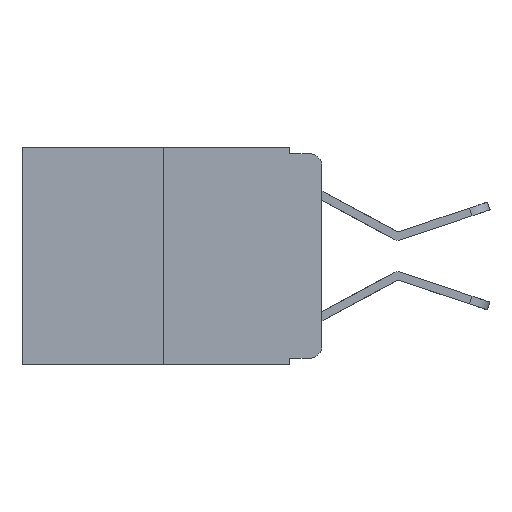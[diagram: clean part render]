
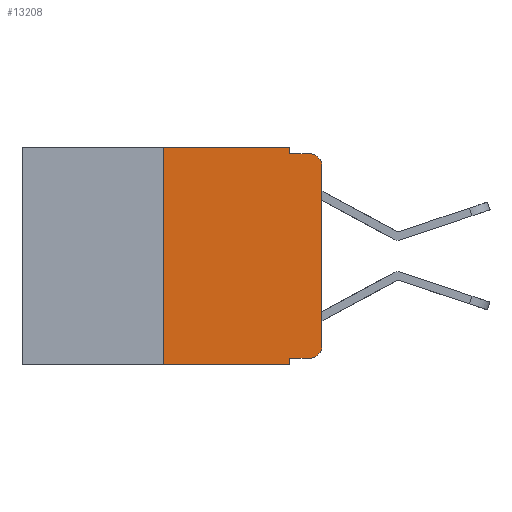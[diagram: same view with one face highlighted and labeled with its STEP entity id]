
A CAD part, left-side view. The second image highlights one B-rep face of the part: STEP entity #13208.
In plain terms, the highlighted planar face has unit normal (-1, 0, 0).
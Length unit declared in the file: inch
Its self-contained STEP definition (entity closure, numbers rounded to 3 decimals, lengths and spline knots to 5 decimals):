
#292 = ORIENTED_EDGE ( 'NONE', *, *, #13894, .F. ) ;
#390 = ORIENTED_EDGE ( 'NONE', *, *, #7782, .F. ) ;
#417 = ORIENTED_EDGE ( 'NONE', *, *, #17921, .T. ) ;
#485 = EDGE_CURVE ( 'NONE', #21264, #4814, #18064, .T. ) ;
#615 = VERTEX_POINT ( 'NONE', #5662 ) ;
#656 = ORIENTED_EDGE ( 'NONE', *, *, #8458, .F. ) ;
#931 = ORIENTED_EDGE ( 'NONE', *, *, #13237, .T. ) ;
#1133 = ORIENTED_EDGE ( 'NONE', *, *, #14154, .T. ) ;
#1221 = CARTESIAN_POINT ( 'NONE',  ( 0., 0.051, 0. ) ) ;
#1790 = AXIS2_PLACEMENT_3D ( 'NONE', #21017, #22693, #12442 ) ;
#2710 = CARTESIAN_POINT ( 'NONE',  ( 0., 0.051, -0.333 ) ) ;
#2815 = DIRECTION ( 'NONE',  ( 0., 0., -1. ) ) ;
#2845 = CARTESIAN_POINT ( 'NONE',  ( 0., 0., 0. ) ) ;
#3142 = CARTESIAN_POINT ( 'NONE',  ( 0., 0.02, -0.01 ) ) ;
#3292 = VERTEX_POINT ( 'NONE', #4111 ) ;
#3741 = ORIENTED_EDGE ( 'NONE', *, *, #21309, .F. ) ;
#4111 = CARTESIAN_POINT ( 'NONE',  ( 0., 0.25, -0.343 ) ) ;
#4673 = VECTOR ( 'NONE', #13669, 39.37008 ) ;
#4814 = VERTEX_POINT ( 'NONE', #3142 ) ;
#4934 = VECTOR ( 'NONE', #2815, 39.37008 ) ;
#5662 = CARTESIAN_POINT ( 'NONE',  ( 0., 0., -0.313 ) ) ;
#5788 = CARTESIAN_POINT ( 'NONE',  ( 0., 0.02, -0.313 ) ) ;
#6361 = DIRECTION ( 'NONE',  ( 0., -1., 0. ) ) ;
#6929 = CARTESIAN_POINT ( 'NONE',  ( 0., 0.473, 0. ) ) ;
#7193 = DIRECTION ( 'NONE',  ( 0., -1., 0. ) ) ;
#7644 = DIRECTION ( 'NONE',  ( 0., 0., -1. ) ) ;
#7782 = EDGE_CURVE ( 'NONE', #3292, #18801, #13699, .T. ) ;
#7798 = EDGE_CURVE ( 'NONE', #615, #21264, #18338, .T. ) ;
#7986 = DIRECTION ( 'NONE',  ( 0., -1., 0. ) ) ;
#8189 = CARTESIAN_POINT ( 'NONE',  ( 0., 0.051, -0.01 ) ) ;
#8267 = CARTESIAN_POINT ( 'NONE',  ( 0., 0.051, -0.343 ) ) ;
#8458 = EDGE_CURVE ( 'NONE', #9088, #21782, #14505, .T. ) ;
#8964 = VECTOR ( 'NONE', #10072, 39.37008 ) ;
#9088 = VERTEX_POINT ( 'NONE', #2710 ) ;
#9343 = LINE ( 'NONE', #6929, #14102 ) ;
#10072 = DIRECTION ( 'NONE',  ( 0., 0., 1. ) ) ;
#10136 = EDGE_LOOP ( 'NONE', ( #10571, #11390, #13653, #3741, #292, #390, #417, #656, #931, #1133 ) ) ;
#10571 = ORIENTED_EDGE ( 'NONE', *, *, #7798, .T. ) ;
#10732 = LINE ( 'NONE', #1221, #19480 ) ;
#11081 = DIRECTION ( 'NONE',  ( 0., 0., -1. ) ) ;
#11182 = VECTOR ( 'NONE', #7986, 39.37008 ) ;
#11390 = ORIENTED_EDGE ( 'NONE', *, *, #485, .T. ) ;
#11472 = AXIS2_PLACEMENT_3D ( 'NONE', #12650, #12436, #11081 ) ;
#11792 = CARTESIAN_POINT ( 'NONE',  ( 0., 0.051, -0.01 ) ) ;
#12303 = LINE ( 'NONE', #16914, #11182 ) ;
#12436 = DIRECTION ( 'NONE',  ( -1., 0., 0. ) ) ;
#12442 = DIRECTION ( 'NONE',  ( 0., 0., -1. ) ) ;
#12650 = CARTESIAN_POINT ( 'NONE',  ( 0., 0.02, -0.03 ) ) ;
#13208 = ADVANCED_FACE ( 'NONE', ( #18477 ), #17669, .F. ) ;
#13237 = EDGE_CURVE ( 'NONE', #9088, #16056, #13295, .T. ) ;
#13295 = LINE ( 'NONE', #17827, #21876 ) ;
#13653 = ORIENTED_EDGE ( 'NONE', *, *, #22832, .F. ) ;
#13669 = DIRECTION ( 'NONE',  ( 0., 0., 1. ) ) ;
#13699 = LINE ( 'NONE', #17147, #8964 ) ;
#13894 = EDGE_CURVE ( 'NONE', #18801, #21827, #9343, .T. ) ;
#14102 = VECTOR ( 'NONE', #19248, 39.37008 ) ;
#14154 = EDGE_CURVE ( 'NONE', #16056, #615, #21836, .T. ) ;
#14505 = LINE ( 'NONE', #15449, #4934 ) ;
#15449 = CARTESIAN_POINT ( 'NONE',  ( 0., 0.051, 0. ) ) ;
#16056 = VERTEX_POINT ( 'NONE', #18286 ) ;
#16694 = VERTEX_POINT ( 'NONE', #8189 ) ;
#16914 = CARTESIAN_POINT ( 'NONE',  ( 0., 0.473, -0.343 ) ) ;
#17147 = CARTESIAN_POINT ( 'NONE',  ( 0., 0.25, 0. ) ) ;
#17424 = DIRECTION ( 'NONE',  ( 0., 0., -1. ) ) ;
#17669 = PLANE ( 'NONE',  #1790 ) ;
#17827 = CARTESIAN_POINT ( 'NONE',  ( 0., 0.051, -0.333 ) ) ;
#17884 = LINE ( 'NONE', #11792, #22294 ) ;
#17921 = EDGE_CURVE ( 'NONE', #3292, #21782, #12303, .T. ) ;
#18064 = CIRCLE ( 'NONE', #11472, 0.02 ) ;
#18212 = DIRECTION ( 'NONE',  ( -1., 0., 0. ) ) ;
#18286 = CARTESIAN_POINT ( 'NONE',  ( 0., 0.02, -0.333 ) ) ;
#18338 = LINE ( 'NONE', #2845, #4673 ) ;
#18477 = FACE_OUTER_BOUND ( 'NONE', #10136, .T. ) ;
#18801 = VERTEX_POINT ( 'NONE', #21420 ) ;
#18871 = CARTESIAN_POINT ( 'NONE',  ( 0., 0.051, 0. ) ) ;
#18893 = CARTESIAN_POINT ( 'NONE',  ( 0., 0., -0.03 ) ) ;
#19248 = DIRECTION ( 'NONE',  ( 0., -1., 0. ) ) ;
#19480 = VECTOR ( 'NONE', #17424, 39.37008 ) ;
#21017 = CARTESIAN_POINT ( 'NONE',  ( 0., 0.473, 0. ) ) ;
#21264 = VERTEX_POINT ( 'NONE', #18893 ) ;
#21309 = EDGE_CURVE ( 'NONE', #21827, #16694, #10732, .T. ) ;
#21420 = CARTESIAN_POINT ( 'NONE',  ( 0., 0.25, 0. ) ) ;
#21782 = VERTEX_POINT ( 'NONE', #8267 ) ;
#21827 = VERTEX_POINT ( 'NONE', #18871 ) ;
#21836 = CIRCLE ( 'NONE', #22216, 0.02 ) ;
#21876 = VECTOR ( 'NONE', #7193, 39.37008 ) ;
#22216 = AXIS2_PLACEMENT_3D ( 'NONE', #5788, #18212, #7644 ) ;
#22294 = VECTOR ( 'NONE', #6361, 39.37008 ) ;
#22693 = DIRECTION ( 'NONE',  ( 1., 0., 0. ) ) ;
#22832 = EDGE_CURVE ( 'NONE', #16694, #4814, #17884, .T. ) ;
